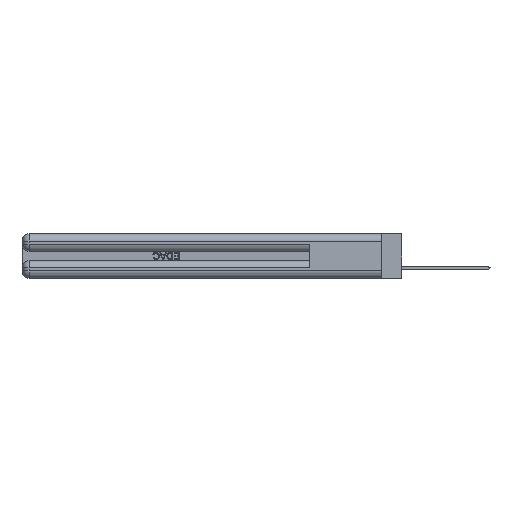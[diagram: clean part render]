
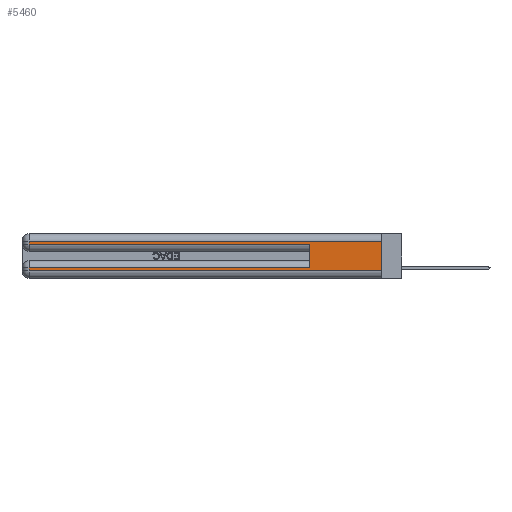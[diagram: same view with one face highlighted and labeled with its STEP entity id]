
A CAD part, left-side view. The second image highlights one B-rep face of the part: STEP entity #5460.
In plain terms, the highlighted planar face has unit normal (-1, 0, 0).
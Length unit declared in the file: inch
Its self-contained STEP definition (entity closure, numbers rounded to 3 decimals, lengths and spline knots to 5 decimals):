
#61 = ORIENTED_EDGE ( 'NONE', *, *, #41126, .T. ) ;
#324 = DIRECTION ( 'NONE',  ( 0., 1., 0. ) ) ;
#380 = VERTEX_POINT ( 'NONE', #35122 ) ;
#1077 = CARTESIAN_POINT ( 'NONE',  ( 0., 0., 0.31 ) ) ;
#1740 = CARTESIAN_POINT ( 'NONE',  ( 0., 0., 0.06 ) ) ;
#1867 = DIRECTION ( 'NONE',  ( 0., 0., -1. ) ) ;
#1948 = FACE_OUTER_BOUND ( 'NONE', #7795, .T. ) ;
#2492 = VECTOR ( 'NONE', #21658, 39.37008 ) ;
#4364 = ORIENTED_EDGE ( 'NONE', *, *, #5870, .T. ) ;
#5125 = CARTESIAN_POINT ( 'NONE',  ( 0., 0., 0.06 ) ) ;
#5460 = ADVANCED_FACE ( 'NONE', ( #1948 ), #20777, .F. ) ;
#5870 = EDGE_CURVE ( 'NONE', #19767, #18931, #31581, .T. ) ;
#6826 = DIRECTION ( 'NONE',  ( 0., -1., 0. ) ) ;
#7476 = VERTEX_POINT ( 'NONE', #8584 ) ;
#7795 = EDGE_LOOP ( 'NONE', ( #38880, #61, #20810, #25123, #39850, #21813, #33161, #4364 ) ) ;
#8213 = LINE ( 'NONE', #36041, #14741 ) ;
#8411 = DIRECTION ( 'NONE',  ( 0., -1., 0. ) ) ;
#8584 = CARTESIAN_POINT ( 'NONE',  ( 0., 0.6, 0.285 ) ) ;
#8770 = LINE ( 'NONE', #41529, #29764 ) ;
#9424 = EDGE_CURVE ( 'NONE', #38983, #7476, #41174, .T. ) ;
#9871 = VECTOR ( 'NONE', #6826, 39.37008 ) ;
#9994 = LINE ( 'NONE', #31531, #2492 ) ;
#10748 = VECTOR ( 'NONE', #26953, 39.37008 ) ;
#11391 = DIRECTION ( 'NONE',  ( 0., 0., -1. ) ) ;
#12733 = VERTEX_POINT ( 'NONE', #36347 ) ;
#13343 = CARTESIAN_POINT ( 'NONE',  ( 0., 0.6, 0.085 ) ) ;
#14226 = CARTESIAN_POINT ( 'NONE',  ( 0., 2.94, 0.06 ) ) ;
#14741 = VECTOR ( 'NONE', #11391, 39.37008 ) ;
#15250 = DIRECTION ( 'NONE',  ( 0., 0., 1. ) ) ;
#18931 = VERTEX_POINT ( 'NONE', #5125 ) ;
#19616 = VECTOR ( 'NONE', #324, 39.37008 ) ;
#19767 = VERTEX_POINT ( 'NONE', #14226 ) ;
#19818 = LINE ( 'NONE', #31981, #9871 ) ;
#20624 = DIRECTION ( 'NONE',  ( 1., 0., 0. ) ) ;
#20777 = PLANE ( 'NONE',  #34938 ) ;
#20810 = ORIENTED_EDGE ( 'NONE', *, *, #38610, .T. ) ;
#21226 = CARTESIAN_POINT ( 'NONE',  ( 0., 0.6, 0.145 ) ) ;
#21658 = DIRECTION ( 'NONE',  ( 0., 0., -1. ) ) ;
#21684 = LINE ( 'NONE', #32400, #19616 ) ;
#21813 = ORIENTED_EDGE ( 'NONE', *, *, #33436, .T. ) ;
#23956 = VECTOR ( 'NONE', #8411, 39.37008 ) ;
#25123 = ORIENTED_EDGE ( 'NONE', *, *, #33917, .T. ) ;
#26763 = CARTESIAN_POINT ( 'NONE',  ( 0., 2.94, 0.31 ) ) ;
#26953 = DIRECTION ( 'NONE',  ( 0., 1., 0. ) ) ;
#29296 = LINE ( 'NONE', #1077, #10748 ) ;
#29764 = VECTOR ( 'NONE', #31923, 39.37008 ) ;
#30640 = CARTESIAN_POINT ( 'NONE',  ( 0., 0., 0.37 ) ) ;
#31531 = CARTESIAN_POINT ( 'NONE',  ( 0., 2.94, 0.37 ) ) ;
#31581 = LINE ( 'NONE', #1740, #23956 ) ;
#31923 = DIRECTION ( 'NONE',  ( 0., 0., -1. ) ) ;
#31981 = CARTESIAN_POINT ( 'NONE',  ( 0., 0., 0.285 ) ) ;
#32198 = VERTEX_POINT ( 'NONE', #35202 ) ;
#32400 = CARTESIAN_POINT ( 'NONE',  ( 0., 0., 0.085 ) ) ;
#32512 = VECTOR ( 'NONE', #15250, 39.37008 ) ;
#33161 = ORIENTED_EDGE ( 'NONE', *, *, #35730, .T. ) ;
#33436 = EDGE_CURVE ( 'NONE', #38983, #32198, #21684, .T. ) ;
#33917 = EDGE_CURVE ( 'NONE', #380, #7476, #19818, .T. ) ;
#34938 = AXIS2_PLACEMENT_3D ( 'NONE', #30640, #20624, #1867 ) ;
#35122 = CARTESIAN_POINT ( 'NONE',  ( 0., 2.94, 0.285 ) ) ;
#35202 = CARTESIAN_POINT ( 'NONE',  ( 0., 2.94, 0.085 ) ) ;
#35301 = VERTEX_POINT ( 'NONE', #26763 ) ;
#35730 = EDGE_CURVE ( 'NONE', #32198, #19767, #8770, .T. ) ;
#36041 = CARTESIAN_POINT ( 'NONE',  ( 0., 0., 0.37 ) ) ;
#36347 = CARTESIAN_POINT ( 'NONE',  ( 0., 0., 0.31 ) ) ;
#36535 = EDGE_CURVE ( 'NONE', #12733, #18931, #8213, .T. ) ;
#38610 = EDGE_CURVE ( 'NONE', #35301, #380, #9994, .T. ) ;
#38880 = ORIENTED_EDGE ( 'NONE', *, *, #36535, .F. ) ;
#38983 = VERTEX_POINT ( 'NONE', #13343 ) ;
#39850 = ORIENTED_EDGE ( 'NONE', *, *, #9424, .F. ) ;
#41126 = EDGE_CURVE ( 'NONE', #12733, #35301, #29296, .T. ) ;
#41174 = LINE ( 'NONE', #21226, #32512 ) ;
#41529 = CARTESIAN_POINT ( 'NONE',  ( 0., 2.94, 0.37 ) ) ;
